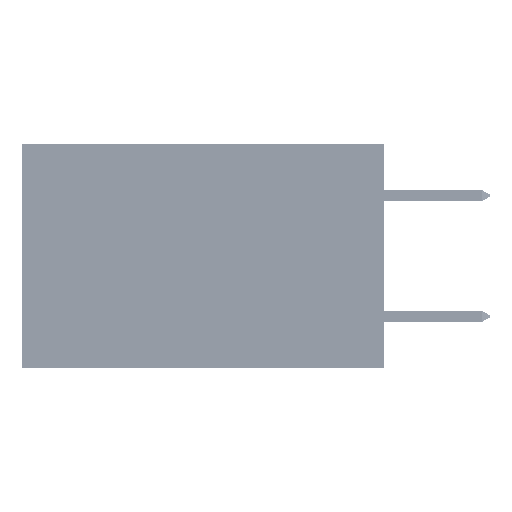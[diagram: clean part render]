
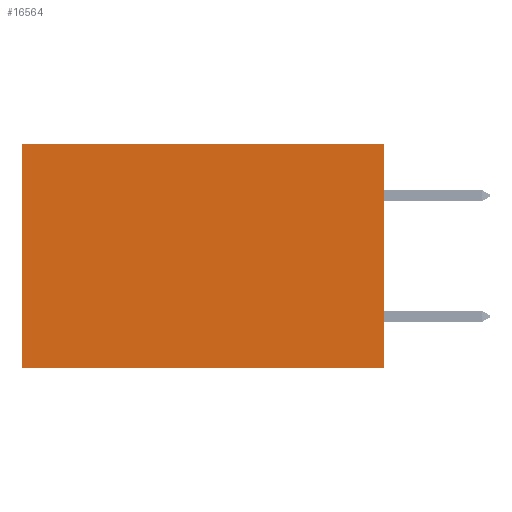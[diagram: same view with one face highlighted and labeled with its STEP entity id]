
A CAD part, left-side view. The second image highlights one B-rep face of the part: STEP entity #16564.
In plain terms, the highlighted planar face has unit normal (-1, 0, 0).
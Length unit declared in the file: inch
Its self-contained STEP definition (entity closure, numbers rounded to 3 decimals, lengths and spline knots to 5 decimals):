
#400 = DIRECTION ( 'NONE',  ( 0., 0., -1. ) ) ;
#2429 = VERTEX_POINT ( 'NONE', #9777 ) ;
#2501 = DIRECTION ( 'NONE',  ( 0., 1., 0. ) ) ;
#4546 = EDGE_CURVE ( 'NONE', #2429, #21104, #23422, .T. ) ;
#5781 = CARTESIAN_POINT ( 'NONE',  ( 0.2875, 0., 0. ) ) ;
#7190 = CARTESIAN_POINT ( 'NONE',  ( 0.2875, 0., -0.37 ) ) ;
#7655 = CARTESIAN_POINT ( 'NONE',  ( 0.2875, 0.6, -0.37 ) ) ;
#7928 = LINE ( 'NONE', #7190, #16094 ) ;
#9777 = CARTESIAN_POINT ( 'NONE',  ( 0.2875, 0., 0. ) ) ;
#10897 = ORIENTED_EDGE ( 'NONE', *, *, #32665, .T. ) ;
#11220 = DIRECTION ( 'NONE',  ( 0., 1., 0. ) ) ;
#15875 = VERTEX_POINT ( 'NONE', #32344 ) ;
#16094 = VECTOR ( 'NONE', #11220, 39.37008 ) ;
#16564 = ADVANCED_FACE ( 'NONE', ( #42197 ), #20361, .F. ) ;
#19549 = VERTEX_POINT ( 'NONE', #7655 ) ;
#20220 = EDGE_LOOP ( 'NONE', ( #51441, #50617, #44066, #10897 ) ) ;
#20244 = LINE ( 'NONE', #26541, #21508 ) ;
#20361 = PLANE ( 'NONE',  #46914 ) ;
#21104 = VERTEX_POINT ( 'NONE', #48403 ) ;
#21508 = VECTOR ( 'NONE', #2501, 39.37008 ) ;
#23422 = LINE ( 'NONE', #5781, #42110 ) ;
#24385 = DIRECTION ( 'NONE',  ( 1., 0., 0. ) ) ;
#25985 = DIRECTION ( 'NONE',  ( 0., 0., -1. ) ) ;
#26541 = CARTESIAN_POINT ( 'NONE',  ( 0.2875, 0., 0. ) ) ;
#27386 = VECTOR ( 'NONE', #35764, 39.37008 ) ;
#28614 = LINE ( 'NONE', #31734, #27386 ) ;
#31734 = CARTESIAN_POINT ( 'NONE',  ( 0.2875, 0.6, 0. ) ) ;
#32344 = CARTESIAN_POINT ( 'NONE',  ( 0.2875, 0.6, 0. ) ) ;
#32665 = EDGE_CURVE ( 'NONE', #2429, #15875, #20244, .T. ) ;
#35764 = DIRECTION ( 'NONE',  ( 0., 0., -1. ) ) ;
#35882 = EDGE_CURVE ( 'NONE', #21104, #19549, #7928, .T. ) ;
#36494 = EDGE_CURVE ( 'NONE', #15875, #19549, #28614, .T. ) ;
#42110 = VECTOR ( 'NONE', #25985, 39.37008 ) ;
#42197 = FACE_OUTER_BOUND ( 'NONE', #20220, .T. ) ;
#44066 = ORIENTED_EDGE ( 'NONE', *, *, #4546, .F. ) ;
#46914 = AXIS2_PLACEMENT_3D ( 'NONE', #48226, #24385, #400 ) ;
#48226 = CARTESIAN_POINT ( 'NONE',  ( 0.2875, 0., 0. ) ) ;
#48403 = CARTESIAN_POINT ( 'NONE',  ( 0.2875, 0., -0.37 ) ) ;
#50617 = ORIENTED_EDGE ( 'NONE', *, *, #35882, .F. ) ;
#51441 = ORIENTED_EDGE ( 'NONE', *, *, #36494, .T. ) ;
